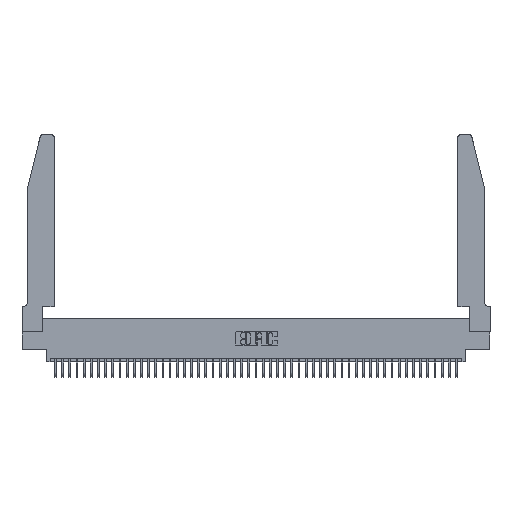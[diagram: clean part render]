
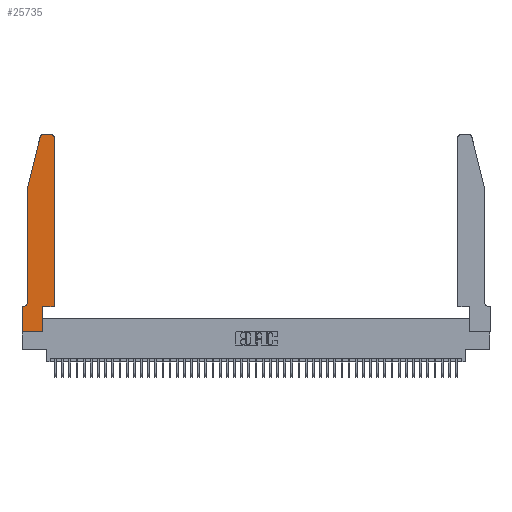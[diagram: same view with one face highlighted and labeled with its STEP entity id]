
A CAD part, top view. The second image highlights one B-rep face of the part: STEP entity #25735.
In plain terms, the highlighted planar face has unit normal (0, 0, 1).
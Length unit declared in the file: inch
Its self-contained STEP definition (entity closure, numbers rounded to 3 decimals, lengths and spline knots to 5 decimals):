
#461 = CARTESIAN_POINT ( 'NONE',  ( 0.0055, 0.35, 0.37 ) ) ;
#518 = DIRECTION ( 'NONE',  ( 1., 0., 0. ) ) ;
#631 = VERTEX_POINT ( 'NONE', #12387 ) ;
#863 = EDGE_CURVE ( 'NONE', #15769, #19052, #16700, .T. ) ;
#1005 = CARTESIAN_POINT ( 'NONE',  ( 0.4505, 2.72, 0.37 ) ) ;
#1479 = VECTOR ( 'NONE', #7676, 39.37008 ) ;
#1747 = DIRECTION ( 'NONE',  ( 0., 1., 0. ) ) ;
#2116 = ORIENTED_EDGE ( 'NONE', *, *, #41308, .T. ) ;
#3047 = ORIENTED_EDGE ( 'NONE', *, *, #41158, .T. ) ;
#4049 = VERTEX_POINT ( 'NONE', #41627 ) ;
#4508 = CARTESIAN_POINT ( 'NONE',  ( 0., 0.35, 0.37 ) ) ;
#5538 = CARTESIAN_POINT ( 'NONE',  ( 0.4205, 2.72, 0.37 ) ) ;
#5680 = VECTOR ( 'NONE', #40879, 39.37008 ) ;
#5724 = DIRECTION ( 'NONE',  ( 0., 1., 0. ) ) ;
#6107 = CARTESIAN_POINT ( 'NONE',  ( 0.0755, 2., 0.37 ) ) ;
#6591 = AXIS2_PLACEMENT_3D ( 'NONE', #26393, #26883, #49243 ) ;
#6631 = ORIENTED_EDGE ( 'NONE', *, *, #863, .T. ) ;
#7393 = VERTEX_POINT ( 'NONE', #461 ) ;
#7676 = DIRECTION ( 'NONE',  ( 1., 0., 0. ) ) ;
#8000 = VERTEX_POINT ( 'NONE', #14171 ) ;
#8691 = CARTESIAN_POINT ( 'NONE',  ( 0., 0., 0.37 ) ) ;
#9362 = CARTESIAN_POINT ( 'NONE',  ( 0.4505, 0.35, 0.37 ) ) ;
#10076 = DIRECTION ( 'NONE',  ( 0., 0., 1. ) ) ;
#10357 = VECTOR ( 'NONE', #1747, 39.37008 ) ;
#10768 = LINE ( 'NONE', #8691, #44671 ) ;
#11651 = LINE ( 'NONE', #45932, #25847 ) ;
#12387 = CARTESIAN_POINT ( 'NONE',  ( 0.2865, 0., 0.37 ) ) ;
#13040 = DIRECTION ( 'NONE',  ( 0., 0., 1. ) ) ;
#13581 = VERTEX_POINT ( 'NONE', #29158 ) ;
#14171 = CARTESIAN_POINT ( 'NONE',  ( 0.0755, 0.42, 0.37 ) ) ;
#14929 = PLANE ( 'NONE',  #31745 ) ;
#15617 = ORIENTED_EDGE ( 'NONE', *, *, #33660, .T. ) ;
#15769 = VERTEX_POINT ( 'NONE', #36100 ) ;
#16163 = ORIENTED_EDGE ( 'NONE', *, *, #41179, .T. ) ;
#16251 = VERTEX_POINT ( 'NONE', #4508 ) ;
#16700 = LINE ( 'NONE', #9362, #34484 ) ;
#17339 = VERTEX_POINT ( 'NONE', #23662 ) ;
#18555 = ORIENTED_EDGE ( 'NONE', *, *, #34261, .T. ) ;
#19052 = VERTEX_POINT ( 'NONE', #1005 ) ;
#20402 = CIRCLE ( 'NONE', #47515, 0.03 ) ;
#21318 = VECTOR ( 'NONE', #30183, 39.37008 ) ;
#21523 = CARTESIAN_POINT ( 'NONE',  ( 0.2865, 0.35, 0.37 ) ) ;
#22116 = EDGE_LOOP ( 'NONE', ( #32844, #26872, #18555, #15617, #3047, #45213, #46963, #35103, #2116, #16163, #6631, #44375 ) ) ;
#22279 = VERTEX_POINT ( 'NONE', #21523 ) ;
#22853 = CIRCLE ( 'NONE', #6591, 0.07 ) ;
#22985 = DIRECTION ( 'NONE',  ( 0., 0., 1. ) ) ;
#23398 = VERTEX_POINT ( 'NONE', #24720 ) ;
#23662 = CARTESIAN_POINT ( 'NONE',  ( 0., 0., 0.37 ) ) ;
#23985 = CARTESIAN_POINT ( 'NONE',  ( 0.0755, 0.35, 0.37 ) ) ;
#24720 = CARTESIAN_POINT ( 'NONE',  ( 0.25487, 2.72718, 0.37 ) ) ;
#25697 = LINE ( 'NONE', #23985, #40596 ) ;
#25735 = ADVANCED_FACE ( 'NONE', ( #43218 ), #14929, .T. ) ;
#25847 = VECTOR ( 'NONE', #38275, 39.37008 ) ;
#26393 = CARTESIAN_POINT ( 'NONE',  ( 0.0055, 0.42, 0.37 ) ) ;
#26872 = ORIENTED_EDGE ( 'NONE', *, *, #28470, .T. ) ;
#26883 = DIRECTION ( 'NONE',  ( 0., 0., -1. ) ) ;
#28317 = VECTOR ( 'NONE', #44146, 39.37008 ) ;
#28470 = EDGE_CURVE ( 'NONE', #13581, #23398, #45386, .T. ) ;
#28809 = EDGE_CURVE ( 'NONE', #7393, #16251, #25697, .T. ) ;
#29158 = CARTESIAN_POINT ( 'NONE',  ( 0.284, 2.75, 0.37 ) ) ;
#30036 = CARTESIAN_POINT ( 'NONE',  ( 0.0755, 2., 0.37 ) ) ;
#30183 = DIRECTION ( 'NONE',  ( -1., 0., 0. ) ) ;
#30592 = LINE ( 'NONE', #30036, #5680 ) ;
#31745 = AXIS2_PLACEMENT_3D ( 'NONE', #45633, #22985, #37965 ) ;
#31778 = DIRECTION ( 'NONE',  ( -1., 0., 0. ) ) ;
#32295 = DIRECTION ( 'NONE',  ( 1., 0., 0. ) ) ;
#32844 = ORIENTED_EDGE ( 'NONE', *, *, #37795, .T. ) ;
#32957 = CARTESIAN_POINT ( 'NONE',  ( 0.284, 2.72, 0.37 ) ) ;
#33660 = EDGE_CURVE ( 'NONE', #4049, #8000, #42601, .T. ) ;
#34261 = EDGE_CURVE ( 'NONE', #23398, #4049, #30592, .T. ) ;
#34484 = VECTOR ( 'NONE', #5724, 39.37008 ) ;
#35103 = ORIENTED_EDGE ( 'NONE', *, *, #36818, .T. ) ;
#35767 = EDGE_CURVE ( 'NONE', #19052, #42026, #20402, .T. ) ;
#36100 = CARTESIAN_POINT ( 'NONE',  ( 0.4505, 0.35, 0.37 ) ) ;
#36205 = LINE ( 'NONE', #37861, #21318 ) ;
#36818 = EDGE_CURVE ( 'NONE', #17339, #631, #10768, .T. ) ;
#37795 = EDGE_CURVE ( 'NONE', #42026, #13581, #36205, .T. ) ;
#37861 = CARTESIAN_POINT ( 'NONE',  ( 0.2605, 2.75, 0.37 ) ) ;
#37965 = DIRECTION ( 'NONE',  ( 1., 0., 0. ) ) ;
#38274 = LINE ( 'NONE', #43458, #10357 ) ;
#38275 = DIRECTION ( 'NONE',  ( 0., -1., 0. ) ) ;
#40596 = VECTOR ( 'NONE', #31778, 39.37008 ) ;
#40598 = EDGE_CURVE ( 'NONE', #16251, #17339, #11651, .T. ) ;
#40879 = DIRECTION ( 'NONE',  ( -0.239, -0.971, 0. ) ) ;
#41158 = EDGE_CURVE ( 'NONE', #8000, #7393, #22853, .T. ) ;
#41179 = EDGE_CURVE ( 'NONE', #22279, #15769, #46073, .T. ) ;
#41308 = EDGE_CURVE ( 'NONE', #631, #22279, #38274, .T. ) ;
#41627 = CARTESIAN_POINT ( 'NONE',  ( 0.0755, 2., 0.37 ) ) ;
#42026 = VERTEX_POINT ( 'NONE', #44630 ) ;
#42069 = DIRECTION ( 'NONE',  ( 1., 0., 0. ) ) ;
#42601 = LINE ( 'NONE', #6107, #28317 ) ;
#43218 = FACE_OUTER_BOUND ( 'NONE', #22116, .T. ) ;
#43458 = CARTESIAN_POINT ( 'NONE',  ( 0.2865, 0.35, 0.37 ) ) ;
#44146 = DIRECTION ( 'NONE',  ( 0., -1., 0. ) ) ;
#44375 = ORIENTED_EDGE ( 'NONE', *, *, #35767, .T. ) ;
#44630 = CARTESIAN_POINT ( 'NONE',  ( 0.4205, 2.75, 0.37 ) ) ;
#44671 = VECTOR ( 'NONE', #42069, 39.37008 ) ;
#45213 = ORIENTED_EDGE ( 'NONE', *, *, #28809, .T. ) ;
#45386 = CIRCLE ( 'NONE', #45829, 0.03 ) ;
#45387 = CARTESIAN_POINT ( 'NONE',  ( 0.4505, 0.35, 0.37 ) ) ;
#45633 = CARTESIAN_POINT ( 'NONE',  ( 0., 0.35, 0.37 ) ) ;
#45829 = AXIS2_PLACEMENT_3D ( 'NONE', #32957, #10076, #32295 ) ;
#45932 = CARTESIAN_POINT ( 'NONE',  ( 0., 0., 0.37 ) ) ;
#46073 = LINE ( 'NONE', #45387, #1479 ) ;
#46963 = ORIENTED_EDGE ( 'NONE', *, *, #40598, .T. ) ;
#47515 = AXIS2_PLACEMENT_3D ( 'NONE', #5538, #13040, #518 ) ;
#49243 = DIRECTION ( 'NONE',  ( -1., 0., 0. ) ) ;
